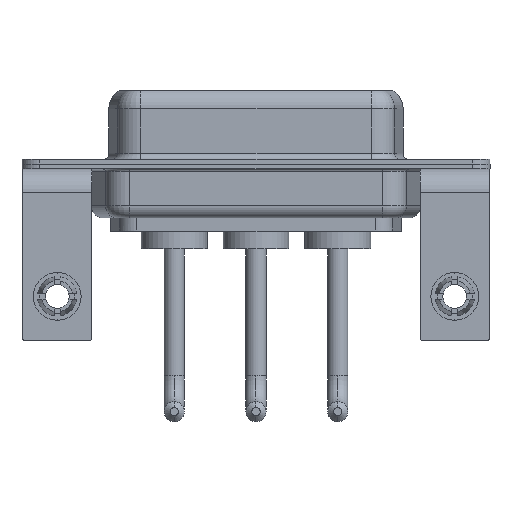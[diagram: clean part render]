
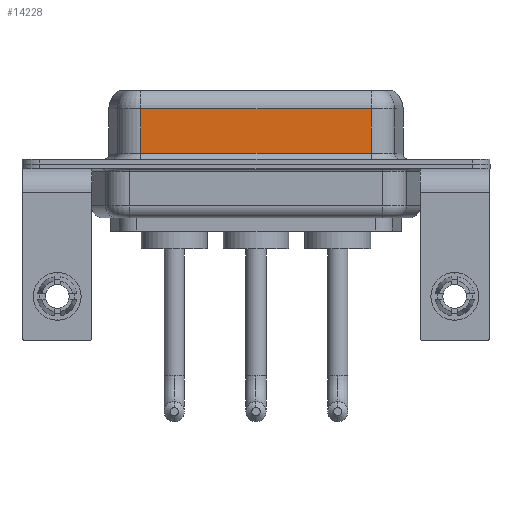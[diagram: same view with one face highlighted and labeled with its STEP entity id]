
A CAD part, front view. The second image highlights one B-rep face of the part: STEP entity #14228.
In plain terms, the highlighted planar face has unit normal (0, -1, 0).
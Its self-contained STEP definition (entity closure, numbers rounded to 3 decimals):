
#13 = CARTESIAN_POINT ( 'NONE',  ( 26.287, -3.95, 4.65 ) ) ;
#130 = AXIS2_PLACEMENT_3D ( 'NONE', #9442, #369, #1574 ) ;
#369 = DIRECTION ( 'NONE',  ( 0., 1., 0. ) ) ;
#764 = VERTEX_POINT ( 'NONE', #12754 ) ;
#780 = LINE ( 'NONE', #7403, #11026 ) ;
#1058 = EDGE_LOOP ( 'NONE', ( #13615, #7460, #9246, #5268 ) ) ;
#1574 = DIRECTION ( 'NONE',  ( 0., 0., 1. ) ) ;
#1953 = VECTOR ( 'NONE', #6236, 1000. ) ;
#1982 = LINE ( 'NONE', #12041, #3525 ) ;
#2646 = VERTEX_POINT ( 'NONE', #13 ) ;
#2950 = CARTESIAN_POINT ( 'NONE',  ( 26.287, -3.95, 0.9 ) ) ;
#2966 = DIRECTION ( 'NONE',  ( 0., 0., -1. ) ) ;
#3107 = LINE ( 'NONE', #12188, #1953 ) ;
#3525 = VECTOR ( 'NONE', #2966, 1000. ) ;
#5268 = ORIENTED_EDGE ( 'NONE', *, *, #7091, .T. ) ;
#5995 = VERTEX_POINT ( 'NONE', #2950 ) ;
#6168 = DIRECTION ( 'NONE',  ( 1., 0., 0. ) ) ;
#6236 = DIRECTION ( 'NONE',  ( 0., 0., -1. ) ) ;
#7091 = EDGE_CURVE ( 'NONE', #764, #5995, #11839, .T. ) ;
#7403 = CARTESIAN_POINT ( 'NONE',  ( 26.287, -3.95, 4.65 ) ) ;
#7430 = CARTESIAN_POINT ( 'NONE',  ( 26.287, -3.95, 0.9 ) ) ;
#7460 = ORIENTED_EDGE ( 'NONE', *, *, #12177, .T. ) ;
#7645 = EDGE_CURVE ( 'NONE', #2646, #5995, #1982, .T. ) ;
#8096 = VECTOR ( 'NONE', #6168, 1000. ) ;
#8715 = CARTESIAN_POINT ( 'NONE',  ( 7.013, -3.95, 4.65 ) ) ;
#8905 = EDGE_CURVE ( 'NONE', #11262, #764, #3107, .T. ) ;
#9246 = ORIENTED_EDGE ( 'NONE', *, *, #8905, .T. ) ;
#9442 = CARTESIAN_POINT ( 'NONE',  ( 26.287, -3.95, 6.4 ) ) ;
#10571 = FACE_OUTER_BOUND ( 'NONE', #1058, .T. ) ;
#11026 = VECTOR ( 'NONE', #11965, 1000. ) ;
#11262 = VERTEX_POINT ( 'NONE', #8715 ) ;
#11839 = LINE ( 'NONE', #7430, #8096 ) ;
#11965 = DIRECTION ( 'NONE',  ( -1., 0., 0. ) ) ;
#12041 = CARTESIAN_POINT ( 'NONE',  ( 26.287, -3.95, 6.4 ) ) ;
#12177 = EDGE_CURVE ( 'NONE', #2646, #11262, #780, .T. ) ;
#12188 = CARTESIAN_POINT ( 'NONE',  ( 7.013, -3.95, 6.4 ) ) ;
#12754 = CARTESIAN_POINT ( 'NONE',  ( 7.013, -3.95, 0.9 ) ) ;
#13120 = PLANE ( 'NONE',  #130 ) ;
#13615 = ORIENTED_EDGE ( 'NONE', *, *, #7645, .F. ) ;
#14228 = ADVANCED_FACE ( 'NONE', ( #10571 ), #13120, .F. ) ;
